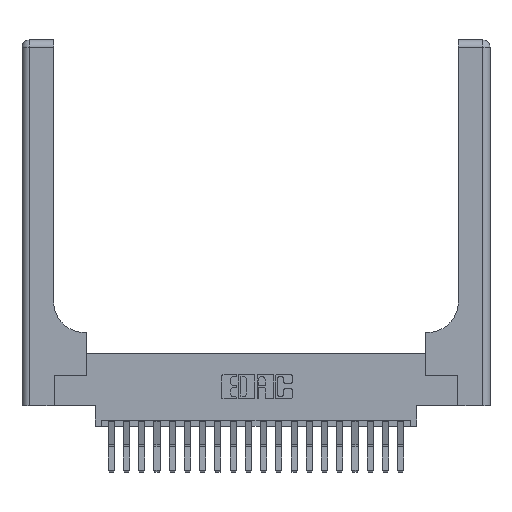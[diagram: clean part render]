
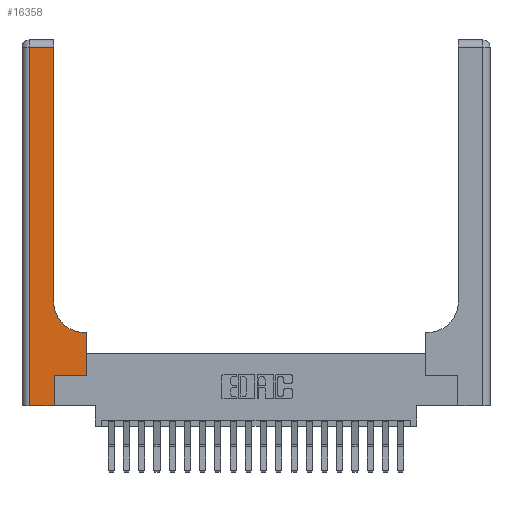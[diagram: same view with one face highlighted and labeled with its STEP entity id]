
A CAD part, top view. The second image highlights one B-rep face of the part: STEP entity #16358.
In plain terms, the highlighted planar face has unit normal (0, 0, 1).
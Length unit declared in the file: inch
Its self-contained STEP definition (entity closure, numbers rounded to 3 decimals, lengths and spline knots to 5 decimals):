
#109 = EDGE_CURVE ( 'NONE', #8870, #1223, #12826, .T. ) ;
#132 = CARTESIAN_POINT ( 'NONE',  ( 0.528, 0.6, 0.37 ) ) ;
#170 = VECTOR ( 'NONE', #10479, 39.37008 ) ;
#268 = ORIENTED_EDGE ( 'NONE', *, *, #18810, .T. ) ;
#806 = DIRECTION ( 'NONE',  ( 0., 1., 0. ) ) ;
#856 = CARTESIAN_POINT ( 'NONE',  ( 0., 2.94, 0.37 ) ) ;
#1101 = CARTESIAN_POINT ( 'NONE',  ( 0., 3., 0.37 ) ) ;
#1223 = VERTEX_POINT ( 'NONE', #11202 ) ;
#1307 = VERTEX_POINT ( 'NONE', #14725 ) ;
#1376 = ORIENTED_EDGE ( 'NONE', *, *, #13197, .T. ) ;
#1678 = DIRECTION ( 'NONE',  ( 1., 0., 0. ) ) ;
#1728 = DIRECTION ( 'NONE',  ( 0., 0., -1. ) ) ;
#1827 = CARTESIAN_POINT ( 'NONE',  ( 0.51, 0.85, 0.37 ) ) ;
#2194 = EDGE_CURVE ( 'NONE', #19937, #2623, #16911, .T. ) ;
#2567 = DIRECTION ( 'NONE',  ( -1., 0., 0. ) ) ;
#2623 = VERTEX_POINT ( 'NONE', #132 ) ;
#2695 = CARTESIAN_POINT ( 'NONE',  ( 0.26, 2.94, 0.37 ) ) ;
#3308 = EDGE_CURVE ( 'NONE', #1223, #15825, #17637, .T. ) ;
#3505 = ORIENTED_EDGE ( 'NONE', *, *, #10867, .T. ) ;
#3542 = VERTEX_POINT ( 'NONE', #6912 ) ;
#3692 = ORIENTED_EDGE ( 'NONE', *, *, #14325, .T. ) ;
#3932 = LINE ( 'NONE', #13279, #16572 ) ;
#4156 = CARTESIAN_POINT ( 'NONE',  ( 0.528, 0.25, 0.37 ) ) ;
#4521 = PLANE ( 'NONE',  #21007 ) ;
#4563 = FACE_OUTER_BOUND ( 'NONE', #8104, .T. ) ;
#4956 = EDGE_CURVE ( 'NONE', #1307, #19937, #9583, .T. ) ;
#5719 = LINE ( 'NONE', #17648, #18338 ) ;
#6076 = VERTEX_POINT ( 'NONE', #18761 ) ;
#6569 = ORIENTED_EDGE ( 'NONE', *, *, #18309, .T. ) ;
#6912 = CARTESIAN_POINT ( 'NONE',  ( 0.265, 0., 0.37 ) ) ;
#7066 = CARTESIAN_POINT ( 'NONE',  ( 0.26, 3., 0.37 ) ) ;
#7203 = DIRECTION ( 'NONE',  ( 1., 0., 0. ) ) ;
#8020 = ORIENTED_EDGE ( 'NONE', *, *, #109, .T. ) ;
#8104 = EDGE_LOOP ( 'NONE', ( #14798, #3692, #6569, #3505, #1376, #11040, #19026, #268, #8020 ) ) ;
#8122 = DIRECTION ( 'NONE',  ( 0., 0., -1. ) ) ;
#8419 = CARTESIAN_POINT ( 'NONE',  ( 0.528, 0.25, 0.37 ) ) ;
#8567 = CARTESIAN_POINT ( 'NONE',  ( 0.06, 3., 0.37 ) ) ;
#8688 = VECTOR ( 'NONE', #806, 39.37008 ) ;
#8870 = VERTEX_POINT ( 'NONE', #11414 ) ;
#8893 = LINE ( 'NONE', #8567, #12726 ) ;
#9583 = LINE ( 'NONE', #18665, #170 ) ;
#10206 = LINE ( 'NONE', #15439, #18435 ) ;
#10479 = DIRECTION ( 'NONE',  ( 1., 0., 0. ) ) ;
#10867 = EDGE_CURVE ( 'NONE', #6076, #3542, #10206, .T. ) ;
#11040 = ORIENTED_EDGE ( 'NONE', *, *, #4956, .T. ) ;
#11202 = CARTESIAN_POINT ( 'NONE',  ( 0.26, 0.85, 0.37 ) ) ;
#11414 = CARTESIAN_POINT ( 'NONE',  ( 0.51, 0.6, 0.37 ) ) ;
#11612 = LINE ( 'NONE', #856, #19829 ) ;
#12726 = VECTOR ( 'NONE', #13523, 39.37008 ) ;
#12826 = CIRCLE ( 'NONE', #18592, 0.25 ) ;
#13197 = EDGE_CURVE ( 'NONE', #3542, #1307, #5719, .T. ) ;
#13279 = CARTESIAN_POINT ( 'NONE',  ( 0.26, 0.6, 0.37 ) ) ;
#13523 = DIRECTION ( 'NONE',  ( 0., -1., 0. ) ) ;
#14325 = EDGE_CURVE ( 'NONE', #15825, #17650, #11612, .T. ) ;
#14342 = DIRECTION ( 'NONE',  ( 0., 1., 0. ) ) ;
#14725 = CARTESIAN_POINT ( 'NONE',  ( 0.265, 0.25, 0.37 ) ) ;
#14798 = ORIENTED_EDGE ( 'NONE', *, *, #3308, .T. ) ;
#14956 = DIRECTION ( 'NONE',  ( -1., 0., 0. ) ) ;
#15439 = CARTESIAN_POINT ( 'NONE',  ( 0., 0., 0.37 ) ) ;
#15825 = VERTEX_POINT ( 'NONE', #2695 ) ;
#16358 = ADVANCED_FACE ( 'NONE', ( #4563 ), #4521, .F. ) ;
#16572 = VECTOR ( 'NONE', #14956, 39.37008 ) ;
#16911 = LINE ( 'NONE', #4156, #8688 ) ;
#16941 = DIRECTION ( 'NONE',  ( 0., 1., 0. ) ) ;
#17128 = VECTOR ( 'NONE', #16941, 39.37008 ) ;
#17637 = LINE ( 'NONE', #7066, #17128 ) ;
#17648 = CARTESIAN_POINT ( 'NONE',  ( 0.265, 0., 0.37 ) ) ;
#17650 = VERTEX_POINT ( 'NONE', #21013 ) ;
#18309 = EDGE_CURVE ( 'NONE', #17650, #6076, #8893, .T. ) ;
#18338 = VECTOR ( 'NONE', #14342, 39.37008 ) ;
#18435 = VECTOR ( 'NONE', #7203, 39.37008 ) ;
#18592 = AXIS2_PLACEMENT_3D ( 'NONE', #1827, #1728, #1678 ) ;
#18665 = CARTESIAN_POINT ( 'NONE',  ( 0.265, 0.25, 0.37 ) ) ;
#18761 = CARTESIAN_POINT ( 'NONE',  ( 0.06, 0., 0.37 ) ) ;
#18810 = EDGE_CURVE ( 'NONE', #2623, #8870, #3932, .T. ) ;
#19026 = ORIENTED_EDGE ( 'NONE', *, *, #2194, .T. ) ;
#19636 = DIRECTION ( 'NONE',  ( -1., 0., 0. ) ) ;
#19829 = VECTOR ( 'NONE', #2567, 39.37008 ) ;
#19937 = VERTEX_POINT ( 'NONE', #8419 ) ;
#21007 = AXIS2_PLACEMENT_3D ( 'NONE', #1101, #8122, #19636 ) ;
#21013 = CARTESIAN_POINT ( 'NONE',  ( 0.06, 2.94, 0.37 ) ) ;
